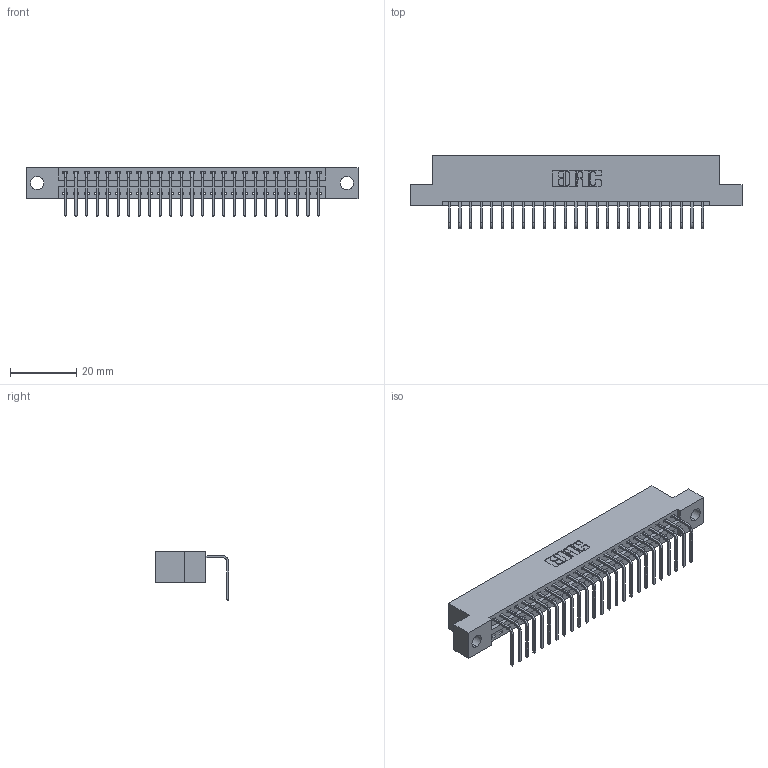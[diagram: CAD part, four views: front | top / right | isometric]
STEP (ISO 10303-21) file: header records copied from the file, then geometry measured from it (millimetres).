
FILE_DESCRIPTION (( 'STEP AP203' ), '1' );
FILE_NAME ('346-025-558-104.STEP', '2022-05-06T01:22:17', ( '' ), ( '' ), 'SwSTEP 2.0', 'SolidWorks 2020', '' );
FILE_SCHEMA (( 'CONFIG_CONTROL_DESIGN' ));
Length unit declared in the file: inch
Products named in the file (3): 346 Part_Flush Mounting Lugs - 0.156 Dia-TH; 346-025-558-104; 345-292-001_558 Tail - 2
Assembly tree (26 placements, depth 2):
  346-025-558-104
    346 Part_Flush Mounting Lugs - 0.156 Dia-TH
    345-292-001_558 Tail - 2  x25
Bounding box: 99.95 x 22.16 x 14.73 mm (x, y, z)
Volume: 9427.5 mm3; surface area: 11933.9 mm2
Topology: 26 solids, 26 shells, 1636 faces, 4915 edges, 3242 vertices
Faces by surface type: plane 1140, cylinder 496
Entity records: 18307 total; most frequent: CARTESIAN_POINT 3153, ORIENTED_EDGE 3110, DIRECTION 2801, EDGE_CURVE 1555, VECTOR 1323, LINE 1323, VERTEX_POINT 1034, AXIS2_PLACEMENT_3D 739
